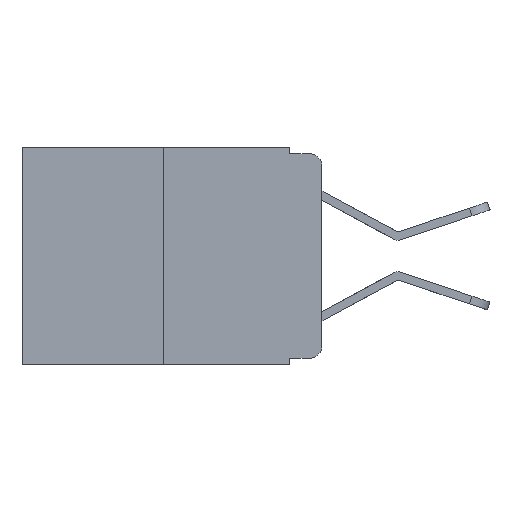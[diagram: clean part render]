
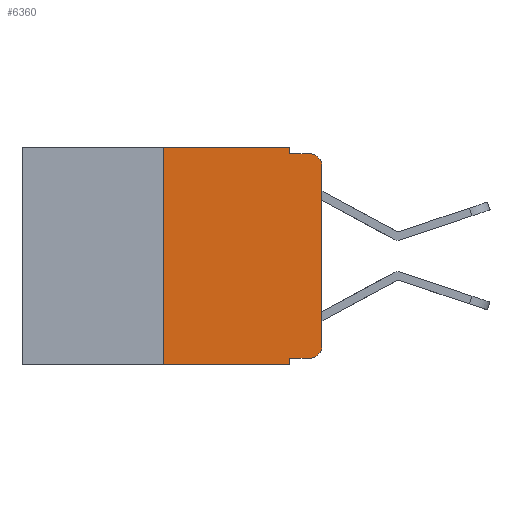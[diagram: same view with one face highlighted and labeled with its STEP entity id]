
A CAD part, left-side view. The second image highlights one B-rep face of the part: STEP entity #6360.
In plain terms, the highlighted planar face has unit normal (-1, 0, 0).
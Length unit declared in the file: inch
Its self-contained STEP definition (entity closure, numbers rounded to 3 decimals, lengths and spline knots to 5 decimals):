
#38 = VECTOR ( 'NONE', #6124, 39.37008 ) ;
#287 = CARTESIAN_POINT ( 'NONE',  ( 0., 0.051, 0. ) ) ;
#507 = LINE ( 'NONE', #7477, #38 ) ;
#639 = AXIS2_PLACEMENT_3D ( 'NONE', #6805, #8508, #14532 ) ;
#922 = EDGE_CURVE ( 'NONE', #7356, #14148, #3704, .T. ) ;
#1019 = VECTOR ( 'NONE', #1950, 39.37008 ) ;
#1028 = EDGE_LOOP ( 'NONE', ( #8886, #3569, #7227, #10436, #12810, #12642, #1171, #15309, #2353, #5824 ) ) ;
#1135 = DIRECTION ( 'NONE',  ( 0., 0., -1. ) ) ;
#1171 = ORIENTED_EDGE ( 'NONE', *, *, #13270, .T. ) ;
#1178 = LINE ( 'NONE', #19899, #13180 ) ;
#1266 = VERTEX_POINT ( 'NONE', #4075 ) ;
#1435 = EDGE_CURVE ( 'NONE', #9544, #7356, #17148, .T. ) ;
#1950 = DIRECTION ( 'NONE',  ( 0., 0., -1. ) ) ;
#2025 = CARTESIAN_POINT ( 'NONE',  ( 0., 0.02, -0.01 ) ) ;
#2285 = VECTOR ( 'NONE', #10746, 39.37008 ) ;
#2353 = ORIENTED_EDGE ( 'NONE', *, *, #6309, .T. ) ;
#2447 = AXIS2_PLACEMENT_3D ( 'NONE', #2995, #18448, #18591 ) ;
#2784 = PLANE ( 'NONE',  #2447 ) ;
#2995 = CARTESIAN_POINT ( 'NONE',  ( 0., 0.473, 0. ) ) ;
#3227 = DIRECTION ( 'NONE',  ( 0., 0., -1. ) ) ;
#3562 = VECTOR ( 'NONE', #9870, 39.37008 ) ;
#3569 = ORIENTED_EDGE ( 'NONE', *, *, #922, .T. ) ;
#3584 = CARTESIAN_POINT ( 'NONE',  ( 0., 0.473, 0. ) ) ;
#3654 = DIRECTION ( 'NONE',  ( 0., 0., 1. ) ) ;
#3704 = CIRCLE ( 'NONE', #18245, 0.02 ) ;
#4075 = CARTESIAN_POINT ( 'NONE',  ( 0., 0.02, -0.333 ) ) ;
#5694 = EDGE_CURVE ( 'NONE', #11324, #14148, #8608, .T. ) ;
#5811 = CARTESIAN_POINT ( 'NONE',  ( 0., 0.051, -0.01 ) ) ;
#5824 = ORIENTED_EDGE ( 'NONE', *, *, #19244, .T. ) ;
#6124 = DIRECTION ( 'NONE',  ( 0., -1., 0. ) ) ;
#6304 = VECTOR ( 'NONE', #3654, 39.37008 ) ;
#6309 = EDGE_CURVE ( 'NONE', #7633, #1266, #507, .T. ) ;
#6360 = ADVANCED_FACE ( 'NONE', ( #9316 ), #2784, .F. ) ;
#6805 = CARTESIAN_POINT ( 'NONE',  ( 0., 0.02, -0.313 ) ) ;
#6826 = CARTESIAN_POINT ( 'NONE',  ( 0., 0.25, -0.343 ) ) ;
#7227 = ORIENTED_EDGE ( 'NONE', *, *, #5694, .F. ) ;
#7356 = VERTEX_POINT ( 'NONE', #14638 ) ;
#7477 = CARTESIAN_POINT ( 'NONE',  ( 0., 0.051, -0.333 ) ) ;
#7633 = VERTEX_POINT ( 'NONE', #18482 ) ;
#8508 = DIRECTION ( 'NONE',  ( -1., 0., 0. ) ) ;
#8608 = LINE ( 'NONE', #5811, #2285 ) ;
#8629 = EDGE_CURVE ( 'NONE', #13672, #14370, #9968, .T. ) ;
#8634 = VERTEX_POINT ( 'NONE', #14727 ) ;
#8886 = ORIENTED_EDGE ( 'NONE', *, *, #1435, .T. ) ;
#8967 = CARTESIAN_POINT ( 'NONE',  ( 0., 0.051, -0.01 ) ) ;
#9184 = LINE ( 'NONE', #3584, #3562 ) ;
#9198 = CARTESIAN_POINT ( 'NONE',  ( 0., 0., 0. ) ) ;
#9316 = FACE_OUTER_BOUND ( 'NONE', #1028, .T. ) ;
#9544 = VERTEX_POINT ( 'NONE', #14999 ) ;
#9581 = LINE ( 'NONE', #287, #1019 ) ;
#9870 = DIRECTION ( 'NONE',  ( 0., -1., 0. ) ) ;
#9905 = EDGE_CURVE ( 'NONE', #14370, #8634, #9184, .T. ) ;
#9968 = LINE ( 'NONE', #17552, #6304 ) ;
#10189 = CARTESIAN_POINT ( 'NONE',  ( 0., 0.051, -0.343 ) ) ;
#10436 = ORIENTED_EDGE ( 'NONE', *, *, #12795, .F. ) ;
#10683 = CIRCLE ( 'NONE', #639, 0.02 ) ;
#10746 = DIRECTION ( 'NONE',  ( 0., -1., 0. ) ) ;
#11324 = VERTEX_POINT ( 'NONE', #8967 ) ;
#12610 = DIRECTION ( 'NONE',  ( -1., 0., 0. ) ) ;
#12642 = ORIENTED_EDGE ( 'NONE', *, *, #8629, .F. ) ;
#12795 = EDGE_CURVE ( 'NONE', #8634, #11324, #1178, .T. ) ;
#12810 = ORIENTED_EDGE ( 'NONE', *, *, #9905, .F. ) ;
#13180 = VECTOR ( 'NONE', #1135, 39.37008 ) ;
#13270 = EDGE_CURVE ( 'NONE', #13672, #15680, #14101, .T. ) ;
#13560 = CARTESIAN_POINT ( 'NONE',  ( 0., 0.473, -0.343 ) ) ;
#13672 = VERTEX_POINT ( 'NONE', #6826 ) ;
#13697 = CARTESIAN_POINT ( 'NONE',  ( 0., 0.25, 0. ) ) ;
#14101 = LINE ( 'NONE', #13560, #16321 ) ;
#14148 = VERTEX_POINT ( 'NONE', #2025 ) ;
#14370 = VERTEX_POINT ( 'NONE', #13697 ) ;
#14532 = DIRECTION ( 'NONE',  ( 0., 0., -1. ) ) ;
#14638 = CARTESIAN_POINT ( 'NONE',  ( 0., 0., -0.03 ) ) ;
#14727 = CARTESIAN_POINT ( 'NONE',  ( 0., 0.051, 0. ) ) ;
#14999 = CARTESIAN_POINT ( 'NONE',  ( 0., 0., -0.313 ) ) ;
#15309 = ORIENTED_EDGE ( 'NONE', *, *, #16631, .F. ) ;
#15680 = VERTEX_POINT ( 'NONE', #10189 ) ;
#16321 = VECTOR ( 'NONE', #18094, 39.37008 ) ;
#16631 = EDGE_CURVE ( 'NONE', #7633, #15680, #9581, .T. ) ;
#17140 = DIRECTION ( 'NONE',  ( 0., 0., 1. ) ) ;
#17148 = LINE ( 'NONE', #9198, #17417 ) ;
#17417 = VECTOR ( 'NONE', #17140, 39.37008 ) ;
#17552 = CARTESIAN_POINT ( 'NONE',  ( 0., 0.25, 0. ) ) ;
#18094 = DIRECTION ( 'NONE',  ( 0., -1., 0. ) ) ;
#18245 = AXIS2_PLACEMENT_3D ( 'NONE', #18952, #12610, #3227 ) ;
#18448 = DIRECTION ( 'NONE',  ( 1., 0., 0. ) ) ;
#18482 = CARTESIAN_POINT ( 'NONE',  ( 0., 0.051, -0.333 ) ) ;
#18591 = DIRECTION ( 'NONE',  ( 0., 0., -1. ) ) ;
#18952 = CARTESIAN_POINT ( 'NONE',  ( 0., 0.02, -0.03 ) ) ;
#19244 = EDGE_CURVE ( 'NONE', #1266, #9544, #10683, .T. ) ;
#19899 = CARTESIAN_POINT ( 'NONE',  ( 0., 0.051, 0. ) ) ;
